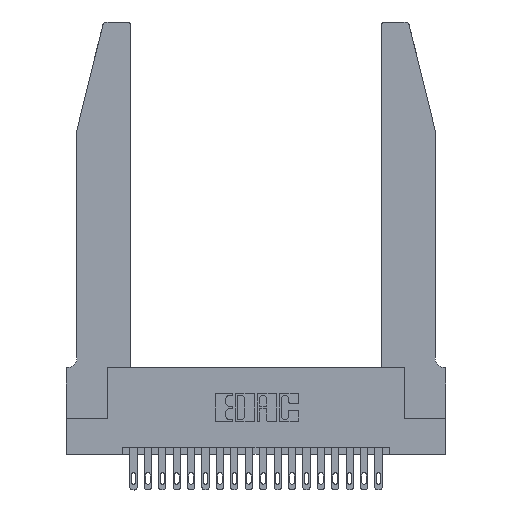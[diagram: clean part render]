
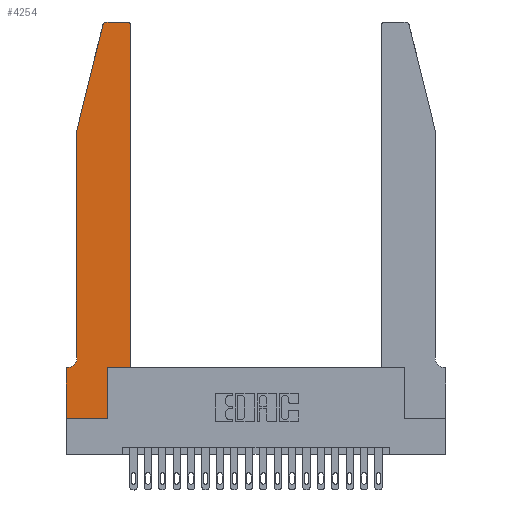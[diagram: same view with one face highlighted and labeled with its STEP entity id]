
A CAD part, top view. The second image highlights one B-rep face of the part: STEP entity #4254.
In plain terms, the highlighted planar face has unit normal (0, 0, 1).
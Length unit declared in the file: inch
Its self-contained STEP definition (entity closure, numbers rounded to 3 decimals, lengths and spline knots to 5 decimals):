
#64 = CARTESIAN_POINT ( 'NONE',  ( 0.4205, 2.72, 0.37 ) ) ;
#136 = VECTOR ( 'NONE', #3319, 39.37008 ) ;
#215 = DIRECTION ( 'NONE',  ( 0., 0., 1. ) ) ;
#265 = EDGE_CURVE ( 'NONE', #6906, #6154, #19195, .T. ) ;
#556 = VERTEX_POINT ( 'NONE', #2479 ) ;
#815 = CARTESIAN_POINT ( 'NONE',  ( 0.4505, 0.35, 0.37 ) ) ;
#833 = CARTESIAN_POINT ( 'NONE',  ( 0.284, 2.75, 0.37 ) ) ;
#897 = DIRECTION ( 'NONE',  ( 1., 0., 0. ) ) ;
#916 = LINE ( 'NONE', #20824, #7323 ) ;
#1196 = ORIENTED_EDGE ( 'NONE', *, *, #12377, .T. ) ;
#1463 = CARTESIAN_POINT ( 'NONE',  ( 0.4505, 0.35, 0.37 ) ) ;
#2479 = CARTESIAN_POINT ( 'NONE',  ( 0.4505, 2.72, 0.37 ) ) ;
#3059 = ORIENTED_EDGE ( 'NONE', *, *, #15711, .T. ) ;
#3071 = LINE ( 'NONE', #17332, #4391 ) ;
#3319 = DIRECTION ( 'NONE',  ( 0., 1., 0. ) ) ;
#3583 = EDGE_CURVE ( 'NONE', #18845, #11213, #14749, .T. ) ;
#3586 = CIRCLE ( 'NONE', #21033, 0.03 ) ;
#3632 = VECTOR ( 'NONE', #11447, 39.37008 ) ;
#3703 = ORIENTED_EDGE ( 'NONE', *, *, #265, .T. ) ;
#4094 = DIRECTION ( 'NONE',  ( 1., 0., 0. ) ) ;
#4096 = ORIENTED_EDGE ( 'NONE', *, *, #15974, .T. ) ;
#4244 = CARTESIAN_POINT ( 'NONE',  ( 0.284, 2.72, 0.37 ) ) ;
#4254 = ADVANCED_FACE ( 'NONE', ( #5928 ), #5873, .T. ) ;
#4385 = CARTESIAN_POINT ( 'NONE',  ( 0., 0.35, 0.37 ) ) ;
#4391 = VECTOR ( 'NONE', #5582, 39.37008 ) ;
#4496 = VECTOR ( 'NONE', #15331, 39.37008 ) ;
#4617 = DIRECTION ( 'NONE',  ( -1., 0., 0. ) ) ;
#4651 = LINE ( 'NONE', #15129, #136 ) ;
#4792 = CARTESIAN_POINT ( 'NONE',  ( 0.2865, 0.35, 0.37 ) ) ;
#4921 = CARTESIAN_POINT ( 'NONE',  ( 0.0755, 2., 0.37 ) ) ;
#5086 = CARTESIAN_POINT ( 'NONE',  ( 0.0755, 2., 0.37 ) ) ;
#5554 = DIRECTION ( 'NONE',  ( 0., 0., -1. ) ) ;
#5582 = DIRECTION ( 'NONE',  ( 0., 1., 0. ) ) ;
#5726 = VECTOR ( 'NONE', #5821, 39.37008 ) ;
#5821 = DIRECTION ( 'NONE',  ( -1., 0., 0. ) ) ;
#5871 = VERTEX_POINT ( 'NONE', #10210 ) ;
#5873 = PLANE ( 'NONE',  #20962 ) ;
#5928 = FACE_OUTER_BOUND ( 'NONE', #20067, .T. ) ;
#6099 = ORIENTED_EDGE ( 'NONE', *, *, #17483, .T. ) ;
#6154 = VERTEX_POINT ( 'NONE', #1463 ) ;
#6157 = EDGE_CURVE ( 'NONE', #15237, #11110, #9590, .T. ) ;
#6906 = VERTEX_POINT ( 'NONE', #4792 ) ;
#7243 = CARTESIAN_POINT ( 'NONE',  ( 0.25487, 2.72718, 0.37 ) ) ;
#7323 = VECTOR ( 'NONE', #20764, 39.37008 ) ;
#7408 = DIRECTION ( 'NONE',  ( -1., 0., 0. ) ) ;
#8272 = VECTOR ( 'NONE', #8295, 39.37008 ) ;
#8295 = DIRECTION ( 'NONE',  ( -0.239, -0.971, 0. ) ) ;
#8788 = AXIS2_PLACEMENT_3D ( 'NONE', #4244, #12836, #897 ) ;
#8861 = LINE ( 'NONE', #13350, #16864 ) ;
#9330 = CARTESIAN_POINT ( 'NONE',  ( 0., 0.35, 0.37 ) ) ;
#9512 = DIRECTION ( 'NONE',  ( 0., 0., 1. ) ) ;
#9589 = VECTOR ( 'NONE', #4094, 39.37008 ) ;
#9590 = LINE ( 'NONE', #5086, #8272 ) ;
#9860 = CIRCLE ( 'NONE', #8788, 0.03 ) ;
#10011 = VERTEX_POINT ( 'NONE', #12864 ) ;
#10105 = CARTESIAN_POINT ( 'NONE',  ( 0.0755, 0.35, 0.37 ) ) ;
#10210 = CARTESIAN_POINT ( 'NONE',  ( 0.0755, 0.42, 0.37 ) ) ;
#10759 = LINE ( 'NONE', #4921, #3632 ) ;
#11074 = ORIENTED_EDGE ( 'NONE', *, *, #13267, .T. ) ;
#11110 = VERTEX_POINT ( 'NONE', #17475 ) ;
#11213 = VERTEX_POINT ( 'NONE', #9330 ) ;
#11447 = DIRECTION ( 'NONE',  ( 0., -1., 0. ) ) ;
#11800 = ORIENTED_EDGE ( 'NONE', *, *, #3583, .T. ) ;
#11939 = DIRECTION ( 'NONE',  ( 1., 0., 0. ) ) ;
#12377 = EDGE_CURVE ( 'NONE', #18533, #15237, #9860, .T. ) ;
#12836 = DIRECTION ( 'NONE',  ( 0., 0., 1. ) ) ;
#12864 = CARTESIAN_POINT ( 'NONE',  ( 0.4205, 2.75, 0.37 ) ) ;
#13267 = EDGE_CURVE ( 'NONE', #5871, #18845, #19170, .T. ) ;
#13350 = CARTESIAN_POINT ( 'NONE',  ( 0.2605, 2.75, 0.37 ) ) ;
#13479 = AXIS2_PLACEMENT_3D ( 'NONE', #17604, #5554, #7408 ) ;
#13752 = CARTESIAN_POINT ( 'NONE',  ( 0., 0., 0.37 ) ) ;
#13850 = EDGE_CURVE ( 'NONE', #11213, #16961, #17551, .T. ) ;
#14727 = ORIENTED_EDGE ( 'NONE', *, *, #19557, .T. ) ;
#14749 = LINE ( 'NONE', #10105, #5726 ) ;
#15129 = CARTESIAN_POINT ( 'NONE',  ( 0.2865, 0.35, 0.37 ) ) ;
#15203 = VERTEX_POINT ( 'NONE', #17304 ) ;
#15237 = VERTEX_POINT ( 'NONE', #7243 ) ;
#15331 = DIRECTION ( 'NONE',  ( 0., -1., 0. ) ) ;
#15444 = ORIENTED_EDGE ( 'NONE', *, *, #6157, .T. ) ;
#15711 = EDGE_CURVE ( 'NONE', #11110, #5871, #10759, .T. ) ;
#15974 = EDGE_CURVE ( 'NONE', #6154, #556, #3071, .T. ) ;
#16270 = DIRECTION ( 'NONE',  ( 1., 0., 0. ) ) ;
#16355 = EDGE_CURVE ( 'NONE', #15203, #6906, #4651, .T. ) ;
#16864 = VECTOR ( 'NONE', #4617, 39.37008 ) ;
#16961 = VERTEX_POINT ( 'NONE', #18188 ) ;
#17304 = CARTESIAN_POINT ( 'NONE',  ( 0.2865, 0., 0.37 ) ) ;
#17332 = CARTESIAN_POINT ( 'NONE',  ( 0.4505, 0.35, 0.37 ) ) ;
#17337 = CARTESIAN_POINT ( 'NONE',  ( 0.0055, 0.35, 0.37 ) ) ;
#17437 = ORIENTED_EDGE ( 'NONE', *, *, #13850, .T. ) ;
#17475 = CARTESIAN_POINT ( 'NONE',  ( 0.0755, 2., 0.37 ) ) ;
#17483 = EDGE_CURVE ( 'NONE', #10011, #18533, #8861, .T. ) ;
#17551 = LINE ( 'NONE', #13752, #4496 ) ;
#17604 = CARTESIAN_POINT ( 'NONE',  ( 0.0055, 0.42, 0.37 ) ) ;
#17903 = ORIENTED_EDGE ( 'NONE', *, *, #19476, .T. ) ;
#18188 = CARTESIAN_POINT ( 'NONE',  ( 0., 0., 0.37 ) ) ;
#18533 = VERTEX_POINT ( 'NONE', #833 ) ;
#18845 = VERTEX_POINT ( 'NONE', #17337 ) ;
#19170 = CIRCLE ( 'NONE', #13479, 0.07 ) ;
#19195 = LINE ( 'NONE', #815, #9589 ) ;
#19476 = EDGE_CURVE ( 'NONE', #556, #10011, #3586, .T. ) ;
#19557 = EDGE_CURVE ( 'NONE', #16961, #15203, #916, .T. ) ;
#20067 = EDGE_LOOP ( 'NONE', ( #6099, #1196, #15444, #3059, #11074, #11800, #17437, #14727, #21651, #3703, #4096, #17903 ) ) ;
#20764 = DIRECTION ( 'NONE',  ( 1., 0., 0. ) ) ;
#20824 = CARTESIAN_POINT ( 'NONE',  ( 0., 0., 0.37 ) ) ;
#20962 = AXIS2_PLACEMENT_3D ( 'NONE', #4385, #9512, #16270 ) ;
#21033 = AXIS2_PLACEMENT_3D ( 'NONE', #64, #215, #11939 ) ;
#21651 = ORIENTED_EDGE ( 'NONE', *, *, #16355, .T. ) ;
